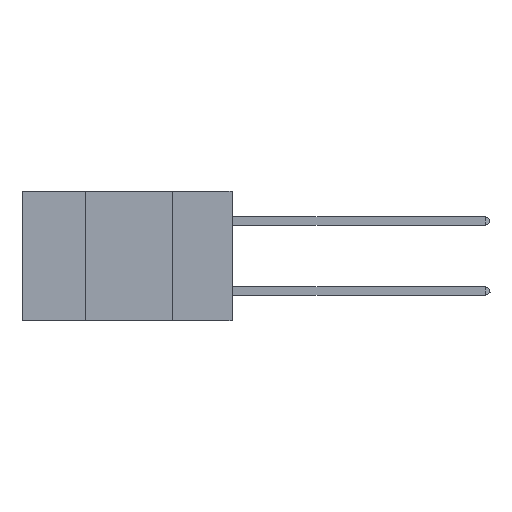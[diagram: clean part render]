
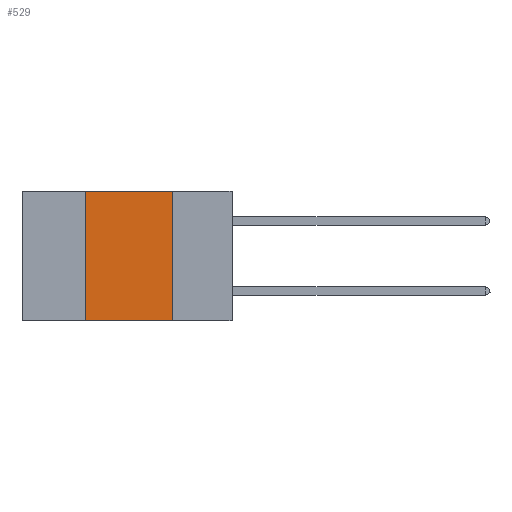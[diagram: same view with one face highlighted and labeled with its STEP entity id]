
A CAD part, left-side view. The second image highlights one B-rep face of the part: STEP entity #529.
In plain terms, the highlighted planar face has unit normal (-1, 0, 0).
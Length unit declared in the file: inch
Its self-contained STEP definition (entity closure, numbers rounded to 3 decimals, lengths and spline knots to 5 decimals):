
#407 = VERTEX_POINT ( 'NONE', #19769 ) ;
#529 = ADVANCED_FACE ( 'NONE', ( #7157 ), #18464, .F. ) ;
#1563 = LINE ( 'NONE', #18408, #17499 ) ;
#2576 = DIRECTION ( 'NONE',  ( 0., -1., 0. ) ) ;
#4449 = DIRECTION ( 'NONE',  ( 0., 0., -1. ) ) ;
#5144 = VERTEX_POINT ( 'NONE', #6793 ) ;
#5644 = EDGE_CURVE ( 'NONE', #8835, #5144, #7369, .T. ) ;
#6001 = EDGE_CURVE ( 'NONE', #5144, #17114, #6134, .T. ) ;
#6134 = LINE ( 'NONE', #10086, #16985 ) ;
#6175 = AXIS2_PLACEMENT_3D ( 'NONE', #10782, #7568, #9198 ) ;
#6793 = CARTESIAN_POINT ( 'NONE',  ( 0., 0.42, 0. ) ) ;
#7157 = FACE_OUTER_BOUND ( 'NONE', #8462, .T. ) ;
#7367 = CARTESIAN_POINT ( 'NONE',  ( 0., 0.42, -0.37 ) ) ;
#7369 = LINE ( 'NONE', #11173, #7855 ) ;
#7519 = EDGE_CURVE ( 'NONE', #17114, #407, #9337, .T. ) ;
#7568 = DIRECTION ( 'NONE',  ( 1., 0., 0. ) ) ;
#7855 = VECTOR ( 'NONE', #17573, 39.37008 ) ;
#8189 = ORIENTED_EDGE ( 'NONE', *, *, #6001, .F. ) ;
#8462 = EDGE_LOOP ( 'NONE', ( #13024, #8189, #17738, #14213 ) ) ;
#8835 = VERTEX_POINT ( 'NONE', #7367 ) ;
#9198 = DIRECTION ( 'NONE',  ( 0., 0., -1. ) ) ;
#9337 = LINE ( 'NONE', #11979, #15691 ) ;
#10086 = CARTESIAN_POINT ( 'NONE',  ( 0., 0.6, 0. ) ) ;
#10782 = CARTESIAN_POINT ( 'NONE',  ( 0., 0.6, 0. ) ) ;
#11173 = CARTESIAN_POINT ( 'NONE',  ( 0., 0.42, 0. ) ) ;
#11979 = CARTESIAN_POINT ( 'NONE',  ( 0., 0.17, 0. ) ) ;
#12432 = DIRECTION ( 'NONE',  ( 0., -1., 0. ) ) ;
#12456 = EDGE_CURVE ( 'NONE', #8835, #407, #1563, .T. ) ;
#13024 = ORIENTED_EDGE ( 'NONE', *, *, #7519, .F. ) ;
#14213 = ORIENTED_EDGE ( 'NONE', *, *, #12456, .T. ) ;
#15691 = VECTOR ( 'NONE', #4449, 39.37008 ) ;
#16909 = CARTESIAN_POINT ( 'NONE',  ( 0., 0.17, 0. ) ) ;
#16985 = VECTOR ( 'NONE', #2576, 39.37008 ) ;
#17114 = VERTEX_POINT ( 'NONE', #16909 ) ;
#17499 = VECTOR ( 'NONE', #12432, 39.37008 ) ;
#17573 = DIRECTION ( 'NONE',  ( 0., 0., 1. ) ) ;
#17738 = ORIENTED_EDGE ( 'NONE', *, *, #5644, .F. ) ;
#18408 = CARTESIAN_POINT ( 'NONE',  ( 0., 0.6, -0.37 ) ) ;
#18464 = PLANE ( 'NONE',  #6175 ) ;
#19769 = CARTESIAN_POINT ( 'NONE',  ( 0., 0.17, -0.37 ) ) ;
